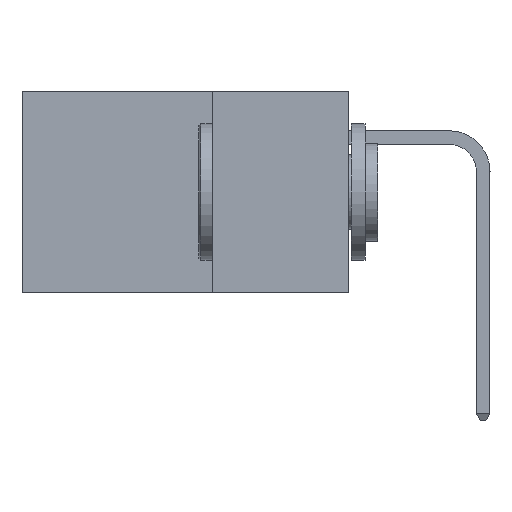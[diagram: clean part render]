
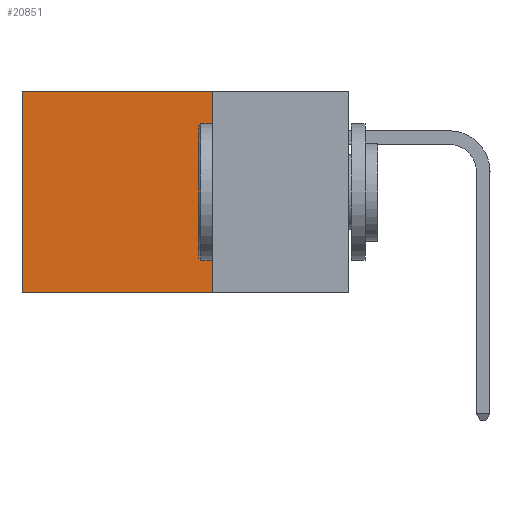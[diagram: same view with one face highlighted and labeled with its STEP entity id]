
A CAD part, left-side view. The second image highlights one B-rep face of the part: STEP entity #20851.
In plain terms, the highlighted planar face has unit normal (-1, 0, 0).
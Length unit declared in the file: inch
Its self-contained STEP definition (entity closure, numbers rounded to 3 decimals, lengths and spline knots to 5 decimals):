
#1615 = EDGE_LOOP ( 'NONE', ( #23112, #28133, #37898, #3217 ) ) ;
#1832 = CARTESIAN_POINT ( 'NONE',  ( 0.2875, 0.25, -0.37 ) ) ;
#2905 = FACE_OUTER_BOUND ( 'NONE', #1615, .T. ) ;
#3217 = ORIENTED_EDGE ( 'NONE', *, *, #22515, .T. ) ;
#4546 = CARTESIAN_POINT ( 'NONE',  ( 0.2875, 0.25, 0. ) ) ;
#5686 = CARTESIAN_POINT ( 'NONE',  ( 0.2875, 0.6, 0. ) ) ;
#6837 = VECTOR ( 'NONE', #32742, 39.37008 ) ;
#9196 = LINE ( 'NONE', #17996, #24445 ) ;
#9545 = VERTEX_POINT ( 'NONE', #32207 ) ;
#9675 = CARTESIAN_POINT ( 'NONE',  ( 0.2875, 0.6, -0.37 ) ) ;
#10890 = PLANE ( 'NONE',  #32371 ) ;
#13048 = VERTEX_POINT ( 'NONE', #27972 ) ;
#15141 = LINE ( 'NONE', #35634, #6837 ) ;
#15950 = CARTESIAN_POINT ( 'NONE',  ( 0.2875, 0.6, 0. ) ) ;
#16025 = VERTEX_POINT ( 'NONE', #5686 ) ;
#17057 = DIRECTION ( 'NONE',  ( 0., 0., -1. ) ) ;
#17339 = DIRECTION ( 'NONE',  ( 0., 1., 0. ) ) ;
#17996 = CARTESIAN_POINT ( 'NONE',  ( 0.2875, 0.25, 0. ) ) ;
#18868 = DIRECTION ( 'NONE',  ( 0., 0., -1. ) ) ;
#20611 = VERTEX_POINT ( 'NONE', #9675 ) ;
#20851 = ADVANCED_FACE ( 'NONE', ( #2905 ), #10890, .F. ) ;
#21128 = VECTOR ( 'NONE', #17339, 39.37008 ) ;
#22515 = EDGE_CURVE ( 'NONE', #9545, #16025, #9196, .T. ) ;
#23112 = ORIENTED_EDGE ( 'NONE', *, *, #27611, .T. ) ;
#24445 = VECTOR ( 'NONE', #33041, 39.37008 ) ;
#25995 = DIRECTION ( 'NONE',  ( 1., 0., 0. ) ) ;
#27325 = EDGE_CURVE ( 'NONE', #9545, #13048, #15141, .T. ) ;
#27611 = EDGE_CURVE ( 'NONE', #16025, #20611, #29725, .T. ) ;
#27972 = CARTESIAN_POINT ( 'NONE',  ( 0.2875, 0.25, -0.37 ) ) ;
#28133 = ORIENTED_EDGE ( 'NONE', *, *, #28554, .F. ) ;
#28554 = EDGE_CURVE ( 'NONE', #13048, #20611, #29142, .T. ) ;
#29142 = LINE ( 'NONE', #1832, #21128 ) ;
#29725 = LINE ( 'NONE', #15950, #38723 ) ;
#32207 = CARTESIAN_POINT ( 'NONE',  ( 0.2875, 0.25, 0. ) ) ;
#32371 = AXIS2_PLACEMENT_3D ( 'NONE', #4546, #25995, #17057 ) ;
#32742 = DIRECTION ( 'NONE',  ( 0., 0., -1. ) ) ;
#33041 = DIRECTION ( 'NONE',  ( 0., 1., 0. ) ) ;
#35634 = CARTESIAN_POINT ( 'NONE',  ( 0.2875, 0.25, 0. ) ) ;
#37898 = ORIENTED_EDGE ( 'NONE', *, *, #27325, .F. ) ;
#38723 = VECTOR ( 'NONE', #18868, 39.37008 ) ;
